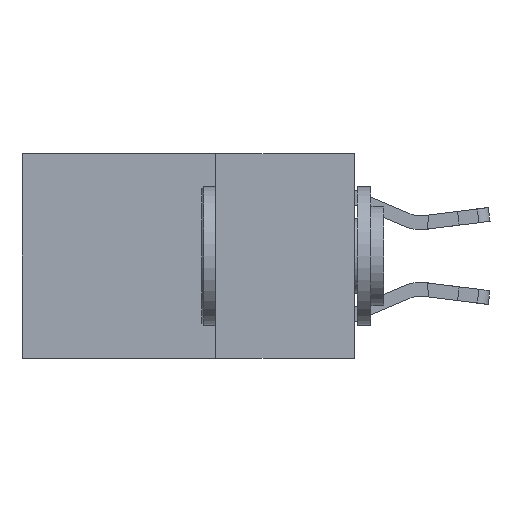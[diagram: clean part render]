
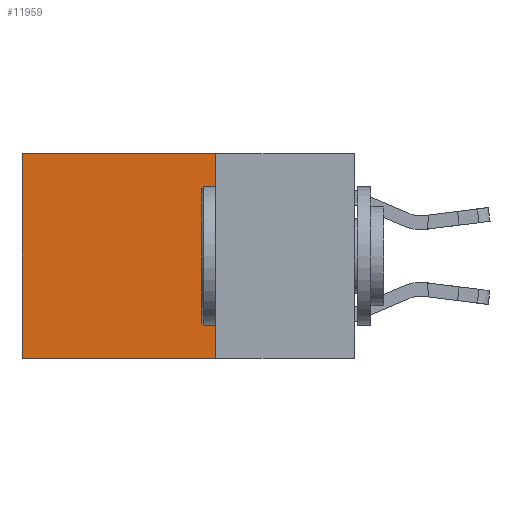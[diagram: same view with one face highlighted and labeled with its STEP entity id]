
A CAD part, left-side view. The second image highlights one B-rep face of the part: STEP entity #11959.
In plain terms, the highlighted planar face has unit normal (-1, 0, 0).
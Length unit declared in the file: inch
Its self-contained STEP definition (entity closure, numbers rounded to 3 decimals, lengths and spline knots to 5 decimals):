
#698 = VECTOR ( 'NONE', #3824, 39.37008 ) ;
#932 = VECTOR ( 'NONE', #1138, 39.37008 ) ;
#1014 = VERTEX_POINT ( 'NONE', #4025 ) ;
#1138 = DIRECTION ( 'NONE',  ( 0., 1., 0. ) ) ;
#1247 = VERTEX_POINT ( 'NONE', #2504 ) ;
#2305 = CARTESIAN_POINT ( 'NONE',  ( 0.2625, 0.25, 0. ) ) ;
#2333 = DIRECTION ( 'NONE',  ( 1., 0., 0. ) ) ;
#2504 = CARTESIAN_POINT ( 'NONE',  ( 0.2625, 0.6, 0. ) ) ;
#3094 = ORIENTED_EDGE ( 'NONE', *, *, #3946, .T. ) ;
#3824 = DIRECTION ( 'NONE',  ( 0., 0., -1. ) ) ;
#3946 = EDGE_CURVE ( 'NONE', #8024, #1247, #8859, .T. ) ;
#4025 = CARTESIAN_POINT ( 'NONE',  ( 0.2625, 0.6, -0.37 ) ) ;
#4778 = CARTESIAN_POINT ( 'NONE',  ( 0.2625, 0.6, 0. ) ) ;
#5009 = LINE ( 'NONE', #10399, #11321 ) ;
#5325 = EDGE_CURVE ( 'NONE', #1247, #1014, #10394, .T. ) ;
#5788 = CARTESIAN_POINT ( 'NONE',  ( 0.2625, 0.25, -0.37 ) ) ;
#6989 = CARTESIAN_POINT ( 'NONE',  ( 0.2625, 0.25, 0. ) ) ;
#7903 = ORIENTED_EDGE ( 'NONE', *, *, #13363, .F. ) ;
#8024 = VERTEX_POINT ( 'NONE', #2305 ) ;
#8438 = ORIENTED_EDGE ( 'NONE', *, *, #5325, .T. ) ;
#8859 = LINE ( 'NONE', #9808, #932 ) ;
#9381 = DIRECTION ( 'NONE',  ( 0., 1., 0. ) ) ;
#9808 = CARTESIAN_POINT ( 'NONE',  ( 0.2625, 0.25, 0. ) ) ;
#9986 = EDGE_CURVE ( 'NONE', #11986, #1014, #5009, .T. ) ;
#10012 = PLANE ( 'NONE',  #13616 ) ;
#10340 = CARTESIAN_POINT ( 'NONE',  ( 0.2625, 0.25, 0. ) ) ;
#10394 = LINE ( 'NONE', #4778, #698 ) ;
#10399 = CARTESIAN_POINT ( 'NONE',  ( 0.2625, 0.25, -0.37 ) ) ;
#11218 = DIRECTION ( 'NONE',  ( 0., 0., -1. ) ) ;
#11321 = VECTOR ( 'NONE', #9381, 39.37008 ) ;
#11617 = LINE ( 'NONE', #10340, #12505 ) ;
#11959 = ADVANCED_FACE ( 'NONE', ( #12020 ), #10012, .F. ) ;
#11986 = VERTEX_POINT ( 'NONE', #5788 ) ;
#12020 = FACE_OUTER_BOUND ( 'NONE', #14086, .T. ) ;
#12505 = VECTOR ( 'NONE', #12619, 39.37008 ) ;
#12619 = DIRECTION ( 'NONE',  ( 0., 0., -1. ) ) ;
#13363 = EDGE_CURVE ( 'NONE', #8024, #11986, #11617, .T. ) ;
#13616 = AXIS2_PLACEMENT_3D ( 'NONE', #6989, #2333, #11218 ) ;
#13827 = ORIENTED_EDGE ( 'NONE', *, *, #9986, .F. ) ;
#14086 = EDGE_LOOP ( 'NONE', ( #8438, #13827, #7903, #3094 ) ) ;
